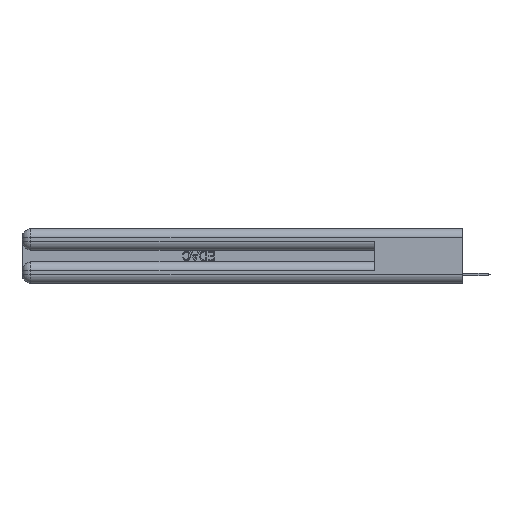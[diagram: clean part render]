
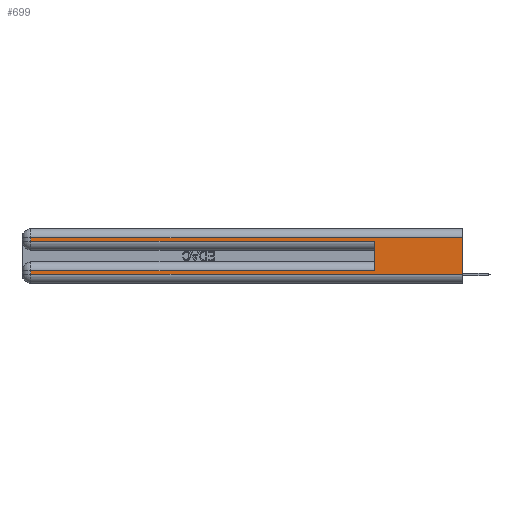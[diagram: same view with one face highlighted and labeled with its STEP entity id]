
A CAD part, left-side view. The second image highlights one B-rep face of the part: STEP entity #699.
In plain terms, the highlighted planar face has unit normal (-1, 0, 0).
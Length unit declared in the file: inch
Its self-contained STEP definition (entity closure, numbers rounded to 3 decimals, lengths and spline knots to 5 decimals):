
#127 = EDGE_CURVE ( 'NONE', #26989, #26113, #9197, .T. ) ;
#699 = ADVANCED_FACE ( 'NONE', ( #15239 ), #8153, .F. ) ;
#807 = CARTESIAN_POINT ( 'NONE',  ( 0., 0.6, 0.085 ) ) ;
#1196 = VERTEX_POINT ( 'NONE', #31566 ) ;
#1449 = VECTOR ( 'NONE', #9059, 39.37008 ) ;
#1498 = LINE ( 'NONE', #28666, #1449 ) ;
#1650 = ORIENTED_EDGE ( 'NONE', *, *, #15230, .T. ) ;
#2130 = CARTESIAN_POINT ( 'NONE',  ( 0., 2.94, 0.37 ) ) ;
#2325 = EDGE_CURVE ( 'NONE', #21706, #23971, #1498, .T. ) ;
#2961 = EDGE_CURVE ( 'NONE', #14016, #23971, #22859, .T. ) ;
#3554 = CARTESIAN_POINT ( 'NONE',  ( 0., 0.6, 0.285 ) ) ;
#4535 = LINE ( 'NONE', #2130, #26309 ) ;
#5011 = CARTESIAN_POINT ( 'NONE',  ( 0., 2.94, 0.37 ) ) ;
#5104 = LINE ( 'NONE', #19904, #7808 ) ;
#5105 = CARTESIAN_POINT ( 'NONE',  ( 0., 0., 0.37 ) ) ;
#6270 = LINE ( 'NONE', #11415, #8244 ) ;
#6743 = DIRECTION ( 'NONE',  ( 0., -1., 0. ) ) ;
#7328 = ORIENTED_EDGE ( 'NONE', *, *, #30220, .T. ) ;
#7808 = VECTOR ( 'NONE', #12170, 39.37008 ) ;
#7860 = VECTOR ( 'NONE', #23700, 39.37008 ) ;
#8153 = PLANE ( 'NONE',  #22650 ) ;
#8244 = VECTOR ( 'NONE', #6743, 39.37008 ) ;
#8667 = ORIENTED_EDGE ( 'NONE', *, *, #127, .F. ) ;
#8817 = CARTESIAN_POINT ( 'NONE',  ( 0., 2.94, 0.285 ) ) ;
#9059 = DIRECTION ( 'NONE',  ( 0., -1., 0. ) ) ;
#9197 = LINE ( 'NONE', #24342, #7860 ) ;
#9223 = LINE ( 'NONE', #24030, #11699 ) ;
#9523 = DIRECTION ( 'NONE',  ( 0., 0., -1. ) ) ;
#10244 = DIRECTION ( 'NONE',  ( 1., 0., 0. ) ) ;
#10300 = DIRECTION ( 'NONE',  ( 0., 0., 1. ) ) ;
#10934 = ORIENTED_EDGE ( 'NONE', *, *, #19986, .T. ) ;
#11415 = CARTESIAN_POINT ( 'NONE',  ( 0., 0., 0.06 ) ) ;
#11699 = VECTOR ( 'NONE', #16467, 39.37008 ) ;
#12073 = CARTESIAN_POINT ( 'NONE',  ( 0., 0., 0.06 ) ) ;
#12170 = DIRECTION ( 'NONE',  ( 0., 1., 0. ) ) ;
#12189 = VERTEX_POINT ( 'NONE', #13622 ) ;
#12314 = CARTESIAN_POINT ( 'NONE',  ( 0., 0., 0.31 ) ) ;
#12406 = DIRECTION ( 'NONE',  ( 0., 0., -1. ) ) ;
#13032 = EDGE_LOOP ( 'NONE', ( #8667, #1650, #10934, #24260, #18554, #14207, #29369, #7328 ) ) ;
#13622 = CARTESIAN_POINT ( 'NONE',  ( 0., 2.94, 0.085 ) ) ;
#14016 = VERTEX_POINT ( 'NONE', #807 ) ;
#14207 = ORIENTED_EDGE ( 'NONE', *, *, #19348, .T. ) ;
#15230 = EDGE_CURVE ( 'NONE', #26989, #1196, #9223, .T. ) ;
#15239 = FACE_OUTER_BOUND ( 'NONE', #13032, .T. ) ;
#16467 = DIRECTION ( 'NONE',  ( 0., 1., 0. ) ) ;
#18554 = ORIENTED_EDGE ( 'NONE', *, *, #2961, .F. ) ;
#18943 = VECTOR ( 'NONE', #10300, 39.37008 ) ;
#19348 = EDGE_CURVE ( 'NONE', #14016, #12189, #5104, .T. ) ;
#19904 = CARTESIAN_POINT ( 'NONE',  ( 0., 0., 0.085 ) ) ;
#19986 = EDGE_CURVE ( 'NONE', #1196, #21706, #4535, .T. ) ;
#21706 = VERTEX_POINT ( 'NONE', #8817 ) ;
#22299 = VECTOR ( 'NONE', #12406, 39.37008 ) ;
#22650 = AXIS2_PLACEMENT_3D ( 'NONE', #5105, #10244, #27625 ) ;
#22859 = LINE ( 'NONE', #25558, #18943 ) ;
#23700 = DIRECTION ( 'NONE',  ( 0., 0., -1. ) ) ;
#23971 = VERTEX_POINT ( 'NONE', #3554 ) ;
#24030 = CARTESIAN_POINT ( 'NONE',  ( 0., 0., 0.31 ) ) ;
#24260 = ORIENTED_EDGE ( 'NONE', *, *, #2325, .T. ) ;
#24342 = CARTESIAN_POINT ( 'NONE',  ( 0., 0., 0.37 ) ) ;
#24417 = VERTEX_POINT ( 'NONE', #24946 ) ;
#24946 = CARTESIAN_POINT ( 'NONE',  ( 0., 2.94, 0.06 ) ) ;
#25558 = CARTESIAN_POINT ( 'NONE',  ( 0., 0.6, 0.145 ) ) ;
#26113 = VERTEX_POINT ( 'NONE', #12073 ) ;
#26309 = VECTOR ( 'NONE', #9523, 39.37008 ) ;
#26989 = VERTEX_POINT ( 'NONE', #12314 ) ;
#27047 = LINE ( 'NONE', #5011, #22299 ) ;
#27625 = DIRECTION ( 'NONE',  ( 0., 0., -1. ) ) ;
#28666 = CARTESIAN_POINT ( 'NONE',  ( 0., 0., 0.285 ) ) ;
#29369 = ORIENTED_EDGE ( 'NONE', *, *, #29909, .T. ) ;
#29909 = EDGE_CURVE ( 'NONE', #12189, #24417, #27047, .T. ) ;
#30220 = EDGE_CURVE ( 'NONE', #24417, #26113, #6270, .T. ) ;
#31566 = CARTESIAN_POINT ( 'NONE',  ( 0., 2.94, 0.31 ) ) ;
